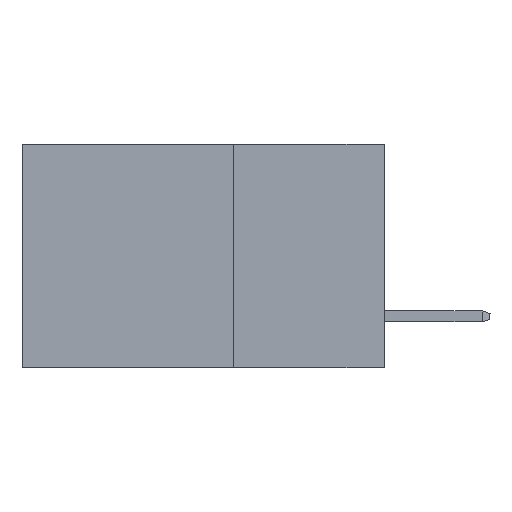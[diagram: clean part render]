
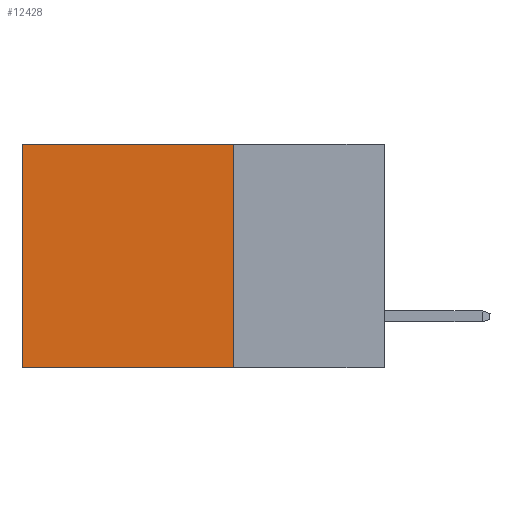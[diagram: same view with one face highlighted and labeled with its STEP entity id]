
A CAD part, left-side view. The second image highlights one B-rep face of the part: STEP entity #12428.
In plain terms, the highlighted planar face has unit normal (-1, 0, 0).
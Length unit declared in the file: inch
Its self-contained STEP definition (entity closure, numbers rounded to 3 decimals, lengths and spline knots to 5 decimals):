
#81 = AXIS2_PLACEMENT_3D ( 'NONE', #3577, #13257, #11780 ) ;
#260 = CARTESIAN_POINT ( 'NONE',  ( 0.298, 0.25, 0. ) ) ;
#394 = DIRECTION ( 'NONE',  ( 0., 1., 0. ) ) ;
#721 = LINE ( 'NONE', #7557, #5271 ) ;
#2151 = FACE_OUTER_BOUND ( 'NONE', #2973, .T. ) ;
#2474 = VECTOR ( 'NONE', #394, 39.37008 ) ;
#2896 = VECTOR ( 'NONE', #11286, 39.37008 ) ;
#2973 = EDGE_LOOP ( 'NONE', ( #5536, #17129, #16770, #7227 ) ) ;
#3247 = EDGE_CURVE ( 'NONE', #5653, #9662, #6143, .T. ) ;
#3520 = LINE ( 'NONE', #13663, #11288 ) ;
#3577 = CARTESIAN_POINT ( 'NONE',  ( 0.298, 0.25, 0. ) ) ;
#3744 = EDGE_CURVE ( 'NONE', #6337, #14412, #3520, .T. ) ;
#3776 = EDGE_CURVE ( 'NONE', #5653, #6337, #5488, .T. ) ;
#5271 = VECTOR ( 'NONE', #17026, 39.37008 ) ;
#5412 = CARTESIAN_POINT ( 'NONE',  ( 0.298, 0.6, -0.37 ) ) ;
#5488 = LINE ( 'NONE', #260, #2896 ) ;
#5536 = ORIENTED_EDGE ( 'NONE', *, *, #6410, .T. ) ;
#5653 = VERTEX_POINT ( 'NONE', #13834 ) ;
#6143 = LINE ( 'NONE', #16687, #2474 ) ;
#6190 = CARTESIAN_POINT ( 'NONE',  ( 0.298, 0.25, -0.37 ) ) ;
#6337 = VERTEX_POINT ( 'NONE', #6190 ) ;
#6410 = EDGE_CURVE ( 'NONE', #9662, #14412, #721, .T. ) ;
#7227 = ORIENTED_EDGE ( 'NONE', *, *, #3247, .T. ) ;
#7557 = CARTESIAN_POINT ( 'NONE',  ( 0.298, 0.6, 0. ) ) ;
#9662 = VERTEX_POINT ( 'NONE', #16095 ) ;
#10975 = DIRECTION ( 'NONE',  ( 0., 1., 0. ) ) ;
#11286 = DIRECTION ( 'NONE',  ( 0., 0., -1. ) ) ;
#11288 = VECTOR ( 'NONE', #10975, 39.37008 ) ;
#11780 = DIRECTION ( 'NONE',  ( 0., 0., -1. ) ) ;
#12428 = ADVANCED_FACE ( 'NONE', ( #2151 ), #15995, .F. ) ;
#13257 = DIRECTION ( 'NONE',  ( 1., 0., 0. ) ) ;
#13663 = CARTESIAN_POINT ( 'NONE',  ( 0.298, 0.25, -0.37 ) ) ;
#13834 = CARTESIAN_POINT ( 'NONE',  ( 0.298, 0.25, 0. ) ) ;
#14412 = VERTEX_POINT ( 'NONE', #5412 ) ;
#15995 = PLANE ( 'NONE',  #81 ) ;
#16095 = CARTESIAN_POINT ( 'NONE',  ( 0.298, 0.6, 0. ) ) ;
#16687 = CARTESIAN_POINT ( 'NONE',  ( 0.298, 0.25, 0. ) ) ;
#16770 = ORIENTED_EDGE ( 'NONE', *, *, #3776, .F. ) ;
#17026 = DIRECTION ( 'NONE',  ( 0., 0., -1. ) ) ;
#17129 = ORIENTED_EDGE ( 'NONE', *, *, #3744, .F. ) ;
